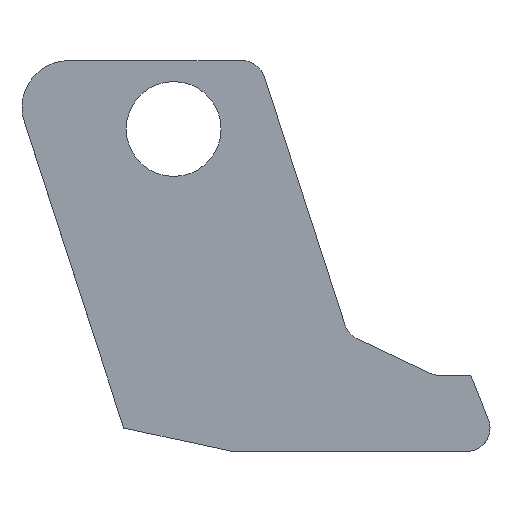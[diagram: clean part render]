
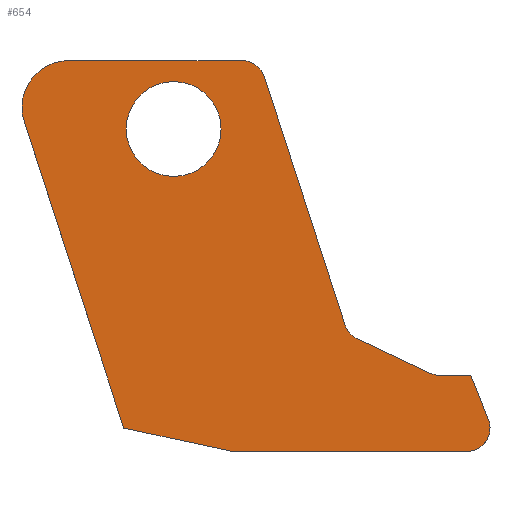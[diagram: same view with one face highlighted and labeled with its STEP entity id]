
A CAD part, front view. The second image highlights one B-rep face of the part: STEP entity #654.
In plain terms, the highlighted planar face has unit normal (0, -1, 0).
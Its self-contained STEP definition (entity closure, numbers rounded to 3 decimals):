
#15=FACE_BOUND('',#79,.T.);
#19=PLANE('',#705);
#43=FACE_OUTER_BOUND('',#78,.T.);
#78=EDGE_LOOP('',(#451,#452,#453,#454,#455,#456,#457,#458,#459,#460,#461,
#462,#463));
#79=EDGE_LOOP('',(#464));
#116=CIRCLE('',#704,1.);
#117=CIRCLE('',#706,1.);
#118=CIRCLE('',#707,1.);
#119=CIRCLE('',#708,1.);
#120=CIRCLE('',#709,2.);
#121=CIRCLE('',#710,2.025);
#140=LINE('',#966,#213);
#141=LINE('',#968,#214);
#142=LINE('',#972,#215);
#143=LINE('',#976,#216);
#144=LINE('',#980,#217);
#145=LINE('',#984,#218);
#146=LINE('',#986,#219);
#147=LINE('',#987,#220);
#213=VECTOR('',#773,10.);
#214=VECTOR('',#774,10.);
#215=VECTOR('',#777,10.);
#216=VECTOR('',#780,10.);
#217=VECTOR('',#783,10.);
#218=VECTOR('',#786,10.);
#219=VECTOR('',#787,10.);
#220=VECTOR('',#788,10.);
#288=VERTEX_POINT('',#959);
#289=VERTEX_POINT('',#961);
#290=VERTEX_POINT('',#965);
#291=VERTEX_POINT('',#967);
#292=VERTEX_POINT('',#969);
#293=VERTEX_POINT('',#971);
#294=VERTEX_POINT('',#973);
#295=VERTEX_POINT('',#975);
#296=VERTEX_POINT('',#977);
#297=VERTEX_POINT('',#979);
#298=VERTEX_POINT('',#981);
#299=VERTEX_POINT('',#983);
#300=VERTEX_POINT('',#985);
#301=VERTEX_POINT('',#988);
#352=EDGE_CURVE('',#288,#289,#116,.T.);
#354=EDGE_CURVE('',#288,#290,#140,.T.);
#355=EDGE_CURVE('',#290,#291,#141,.T.);
#356=EDGE_CURVE('',#292,#291,#117,.T.);
#357=EDGE_CURVE('',#293,#292,#142,.T.);
#358=EDGE_CURVE('',#294,#293,#118,.T.);
#359=EDGE_CURVE('',#295,#294,#143,.T.);
#360=EDGE_CURVE('',#296,#295,#119,.T.);
#361=EDGE_CURVE('',#296,#297,#144,.T.);
#362=EDGE_CURVE('',#298,#297,#120,.T.);
#363=EDGE_CURVE('',#299,#298,#145,.T.);
#364=EDGE_CURVE('',#299,#300,#146,.T.);
#365=EDGE_CURVE('',#289,#300,#147,.T.);
#366=EDGE_CURVE('',#301,#301,#121,.T.);
#451=ORIENTED_EDGE('',*,*,#352,.F.);
#452=ORIENTED_EDGE('',*,*,#354,.T.);
#453=ORIENTED_EDGE('',*,*,#355,.T.);
#454=ORIENTED_EDGE('',*,*,#356,.F.);
#455=ORIENTED_EDGE('',*,*,#357,.F.);
#456=ORIENTED_EDGE('',*,*,#358,.F.);
#457=ORIENTED_EDGE('',*,*,#359,.F.);
#458=ORIENTED_EDGE('',*,*,#360,.F.);
#459=ORIENTED_EDGE('',*,*,#361,.T.);
#460=ORIENTED_EDGE('',*,*,#362,.F.);
#461=ORIENTED_EDGE('',*,*,#363,.F.);
#462=ORIENTED_EDGE('',*,*,#364,.T.);
#463=ORIENTED_EDGE('',*,*,#365,.F.);
#464=ORIENTED_EDGE('',*,*,#366,.F.);
#654=ADVANCED_FACE('',(#43,#15),#19,.F.);
#704=AXIS2_PLACEMENT_3D('',#962,#768,#769);
#705=AXIS2_PLACEMENT_3D('',#964,#771,#772);
#706=AXIS2_PLACEMENT_3D('',#970,#775,#776);
#707=AXIS2_PLACEMENT_3D('',#974,#778,#779);
#708=AXIS2_PLACEMENT_3D('',#978,#781,#782);
#709=AXIS2_PLACEMENT_3D('',#982,#784,#785);
#710=AXIS2_PLACEMENT_3D('',#989,#789,#790);
#768=DIRECTION('center_axis',(0.,1.,0.));
#769=DIRECTION('ref_axis',(0.828,0.,-0.561));
#771=DIRECTION('center_axis',(0.,1.,0.));
#772=DIRECTION('ref_axis',(1.,0.,0.));
#773=DIRECTION('',(-0.371,0.,0.929));
#774=DIRECTION('',(-1.,0.,0.));
#775=DIRECTION('center_axis',(0.,-1.,0.));
#776=DIRECTION('ref_axis',(-0.219,0.,-0.976));
#777=DIRECTION('',(0.904,0.,-0.428));
#778=DIRECTION('center_axis',(0.,-1.,0.));
#779=DIRECTION('ref_axis',(-0.751,0.,-0.66));
#780=DIRECTION('',(0.309,0.,-0.951));
#781=DIRECTION('center_axis',(0.,1.,0.));
#782=DIRECTION('ref_axis',(0.588,0.,0.809));
#783=DIRECTION('',(-1.,0.,0.));
#784=DIRECTION('center_axis',(0.,1.,0.));
#785=DIRECTION('ref_axis',(-0.809,0.,0.588));
#786=DIRECTION('',(-0.309,0.,0.951));
#787=DIRECTION('',(0.978,0.,-0.211));
#788=DIRECTION('',(-1.,0.,0.));
#789=DIRECTION('center_axis',(0.,-1.,0.));
#790=DIRECTION('ref_axis',(1.,0.,0.));
#959=CARTESIAN_POINT('',(13.445,-1.025,-12.404));
#961=CARTESIAN_POINT('',(12.517,-1.025,-13.775));
#962=CARTESIAN_POINT('Origin',(12.517,-1.025,-12.775));
#964=CARTESIAN_POINT('Origin',(3.38,-1.025,-5.425));
#965=CARTESIAN_POINT('',(12.694,-1.025,-10.525));
#966=CARTESIAN_POINT('',(13.993,-1.025,-13.775));
#967=CARTESIAN_POINT('',(11.369,-1.025,-10.525));
#968=CARTESIAN_POINT('',(12.694,-1.025,-10.525));
#969=CARTESIAN_POINT('',(10.941,-1.025,-10.429));
#970=CARTESIAN_POINT('Origin',(11.369,-1.025,-9.525));
#971=CARTESIAN_POINT('',(7.841,-1.025,-8.96));
#972=CARTESIAN_POINT('',(7.451,-1.025,-8.775));
#973=CARTESIAN_POINT('',(7.318,-1.025,-8.365));
#974=CARTESIAN_POINT('Origin',(8.269,-1.025,-8.056));
#975=CARTESIAN_POINT('',(3.874,-1.025,2.234));
#976=CARTESIAN_POINT('',(3.65,-1.025,2.925));
#977=CARTESIAN_POINT('',(2.923,-1.025,2.925));
#978=CARTESIAN_POINT('Origin',(2.923,-1.025,1.925));
#979=CARTESIAN_POINT('',(-4.48,-1.025,2.925));
#980=CARTESIAN_POINT('',(3.65,-1.025,2.925));
#981=CARTESIAN_POINT('',(-6.382,-1.025,0.307));
#982=CARTESIAN_POINT('Origin',(-4.48,-1.025,0.925));
#983=CARTESIAN_POINT('',(-2.132,-1.025,-12.775));
#984=CARTESIAN_POINT('',(-1.807,-1.025,-13.775));
#985=CARTESIAN_POINT('',(2.512,-1.025,-13.775));
#986=CARTESIAN_POINT('',(2.068,-1.025,-13.679));
#987=CARTESIAN_POINT('',(13.993,-1.025,-13.775));
#988=CARTESIAN_POINT('',(-2.025,-1.025,0.));
#989=CARTESIAN_POINT('Origin',(0.,-1.025,0.));
